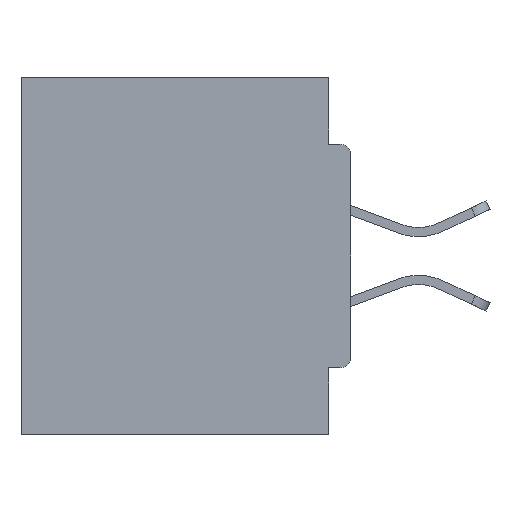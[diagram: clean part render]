
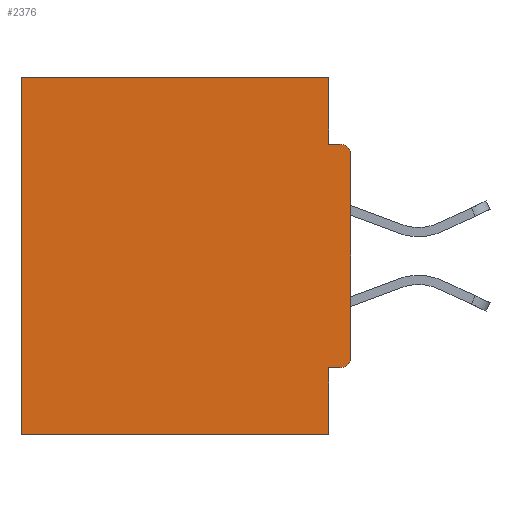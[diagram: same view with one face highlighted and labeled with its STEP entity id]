
A CAD part, left-side view. The second image highlights one B-rep face of the part: STEP entity #2376.
In plain terms, the highlighted planar face has unit normal (-1, 0, 0).
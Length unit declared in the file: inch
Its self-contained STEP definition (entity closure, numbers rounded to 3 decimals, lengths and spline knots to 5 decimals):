
#32 = ORIENTED_EDGE ( 'NONE', *, *, #35251, .T. ) ;
#138 = EDGE_LOOP ( 'NONE', ( #16639, #13571, #19332, #11964, #25084, #21666, #27903, #12551, #32, #12754 ) ) ;
#1102 = VERTEX_POINT ( 'NONE', #6465 ) ;
#1544 = DIRECTION ( 'NONE',  ( 0., 1., 0. ) ) ;
#1957 = EDGE_CURVE ( 'NONE', #7870, #2599, #35074, .T. ) ;
#2163 = CARTESIAN_POINT ( 'NONE',  ( 0.298, 0.015, -0.3915 ) ) ;
#2376 = ADVANCED_FACE ( 'NONE', ( #25684 ), #6497, .F. ) ;
#2599 = VERTEX_POINT ( 'NONE', #14563 ) ;
#4432 = DIRECTION ( 'NONE',  ( 0., 0., -1. ) ) ;
#4599 = DIRECTION ( 'NONE',  ( 0., 0., -1. ) ) ;
#6063 = DIRECTION ( 'NONE',  ( 0., 0., -1. ) ) ;
#6465 = CARTESIAN_POINT ( 'NONE',  ( 0.298, 0.031, -0.5 ) ) ;
#6497 = PLANE ( 'NONE',  #11146 ) ;
#7645 = DIRECTION ( 'NONE',  ( 0., 0., -1. ) ) ;
#7845 = CARTESIAN_POINT ( 'NONE',  ( 0.298, 0.46, -0.5 ) ) ;
#7870 = VERTEX_POINT ( 'NONE', #37381 ) ;
#8693 = VECTOR ( 'NONE', #1544, 39.37008 ) ;
#9496 = DIRECTION ( 'NONE',  ( 1., 0., 0. ) ) ;
#10089 = VERTEX_POINT ( 'NONE', #15348 ) ;
#10542 = EDGE_CURVE ( 'NONE', #7870, #12134, #36044, .T. ) ;
#11146 = AXIS2_PLACEMENT_3D ( 'NONE', #27090, #9496, #15518 ) ;
#11836 = LINE ( 'NONE', #27344, #15599 ) ;
#11964 = ORIENTED_EDGE ( 'NONE', *, *, #16934, .T. ) ;
#12134 = VERTEX_POINT ( 'NONE', #16186 ) ;
#12551 = ORIENTED_EDGE ( 'NONE', *, *, #36364, .F. ) ;
#12754 = ORIENTED_EDGE ( 'NONE', *, *, #10542, .F. ) ;
#13571 = ORIENTED_EDGE ( 'NONE', *, *, #24877, .F. ) ;
#13832 = CARTESIAN_POINT ( 'NONE',  ( 0.298, 0., -0.4065 ) ) ;
#14192 = DIRECTION ( 'NONE',  ( 0., 1., 0. ) ) ;
#14563 = CARTESIAN_POINT ( 'NONE',  ( 0.298, 0.015, -0.0935 ) ) ;
#14753 = VERTEX_POINT ( 'NONE', #28865 ) ;
#14763 = LINE ( 'NONE', #13832, #8693 ) ;
#14769 = EDGE_CURVE ( 'NONE', #23908, #36296, #37748, .T. ) ;
#15023 = VECTOR ( 'NONE', #6063, 39.37008 ) ;
#15348 = CARTESIAN_POINT ( 'NONE',  ( 0.298, 0.015, -0.4065 ) ) ;
#15518 = DIRECTION ( 'NONE',  ( 0., 0., -1. ) ) ;
#15599 = VECTOR ( 'NONE', #27477, 39.37008 ) ;
#15628 = CARTESIAN_POINT ( 'NONE',  ( 0.298, 0.031, -0.4065 ) ) ;
#16186 = CARTESIAN_POINT ( 'NONE',  ( 0.298, 0., -0.3915 ) ) ;
#16639 = ORIENTED_EDGE ( 'NONE', *, *, #1957, .T. ) ;
#16798 = CARTESIAN_POINT ( 'NONE',  ( 0.298, 0., -0.5 ) ) ;
#16934 = EDGE_CURVE ( 'NONE', #23908, #14753, #34331, .T. ) ;
#17387 = LINE ( 'NONE', #26081, #30956 ) ;
#18351 = LINE ( 'NONE', #16798, #36139 ) ;
#18641 = CARTESIAN_POINT ( 'NONE',  ( 0.298, 0.031, -0.0935 ) ) ;
#19168 = DIRECTION ( 'NONE',  ( -1., 0., 0. ) ) ;
#19332 = ORIENTED_EDGE ( 'NONE', *, *, #14769, .F. ) ;
#19637 = LINE ( 'NONE', #31376, #26177 ) ;
#19873 = AXIS2_PLACEMENT_3D ( 'NONE', #22292, #19168, #4432 ) ;
#20000 = DIRECTION ( 'NONE',  ( 0., 1., 0. ) ) ;
#21329 = CARTESIAN_POINT ( 'NONE',  ( 0.298, 0., 0. ) ) ;
#21666 = ORIENTED_EDGE ( 'NONE', *, *, #31631, .F. ) ;
#22292 = CARTESIAN_POINT ( 'NONE',  ( 0.298, 0.015, -0.1085 ) ) ;
#22373 = VERTEX_POINT ( 'NONE', #7845 ) ;
#22689 = DIRECTION ( 'NONE',  ( 0., -1., 0. ) ) ;
#23908 = VERTEX_POINT ( 'NONE', #30992 ) ;
#24877 = EDGE_CURVE ( 'NONE', #36296, #2599, #17387, .T. ) ;
#25084 = ORIENTED_EDGE ( 'NONE', *, *, #36802, .T. ) ;
#25684 = FACE_OUTER_BOUND ( 'NONE', #138, .T. ) ;
#25968 = EDGE_CURVE ( 'NONE', #38660, #1102, #19637, .T. ) ;
#26081 = CARTESIAN_POINT ( 'NONE',  ( 0.298, 0., -0.0935 ) ) ;
#26177 = VECTOR ( 'NONE', #7645, 39.37008 ) ;
#27090 = CARTESIAN_POINT ( 'NONE',  ( 0.298, 0., 0. ) ) ;
#27344 = CARTESIAN_POINT ( 'NONE',  ( 0.298, 0.46, 0. ) ) ;
#27477 = DIRECTION ( 'NONE',  ( 0., 0., -1. ) ) ;
#27903 = ORIENTED_EDGE ( 'NONE', *, *, #25968, .F. ) ;
#28865 = CARTESIAN_POINT ( 'NONE',  ( 0.298, 0.46, 0. ) ) ;
#29149 = CARTESIAN_POINT ( 'NONE',  ( 0.298, 0., 0. ) ) ;
#29300 = DIRECTION ( 'NONE',  ( -1., 0., 0. ) ) ;
#29793 = VECTOR ( 'NONE', #4599, 39.37008 ) ;
#30956 = VECTOR ( 'NONE', #22689, 39.37008 ) ;
#30992 = CARTESIAN_POINT ( 'NONE',  ( 0.298, 0.031, 0. ) ) ;
#31376 = CARTESIAN_POINT ( 'NONE',  ( 0.298, 0.031, -0.5 ) ) ;
#31631 = EDGE_CURVE ( 'NONE', #1102, #22373, #18351, .T. ) ;
#31891 = DIRECTION ( 'NONE',  ( 0., 0., -1. ) ) ;
#34331 = LINE ( 'NONE', #29149, #36661 ) ;
#34403 = CIRCLE ( 'NONE', #35574, 0.015 ) ;
#35074 = CIRCLE ( 'NONE', #19873, 0.015 ) ;
#35251 = EDGE_CURVE ( 'NONE', #10089, #12134, #34403, .T. ) ;
#35574 = AXIS2_PLACEMENT_3D ( 'NONE', #2163, #29300, #31891 ) ;
#36044 = LINE ( 'NONE', #21329, #15023 ) ;
#36139 = VECTOR ( 'NONE', #14192, 39.37008 ) ;
#36296 = VERTEX_POINT ( 'NONE', #18641 ) ;
#36364 = EDGE_CURVE ( 'NONE', #10089, #38660, #14763, .T. ) ;
#36661 = VECTOR ( 'NONE', #20000, 39.37008 ) ;
#36802 = EDGE_CURVE ( 'NONE', #14753, #22373, #11836, .T. ) ;
#37381 = CARTESIAN_POINT ( 'NONE',  ( 0.298, 0., -0.1085 ) ) ;
#37748 = LINE ( 'NONE', #38026, #29793 ) ;
#38026 = CARTESIAN_POINT ( 'NONE',  ( 0.298, 0.031, -0.5 ) ) ;
#38660 = VERTEX_POINT ( 'NONE', #15628 ) ;
